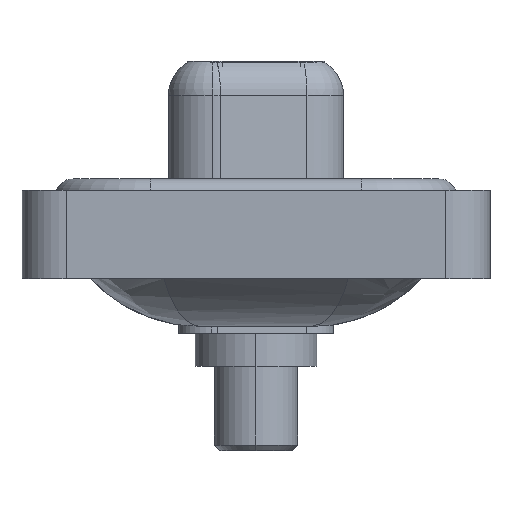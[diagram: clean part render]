
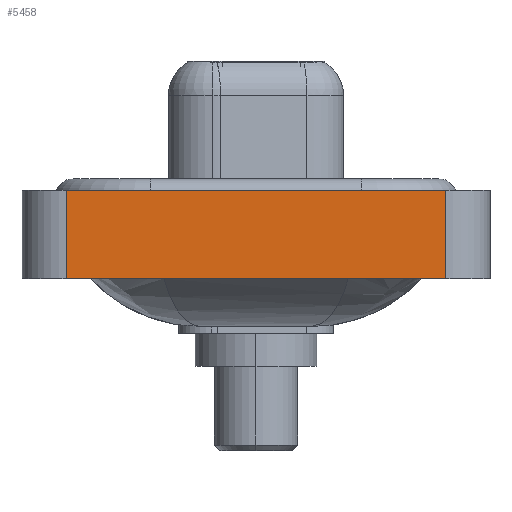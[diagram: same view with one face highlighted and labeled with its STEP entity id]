
A CAD part, left-side view. The second image highlights one B-rep face of the part: STEP entity #5458.
In plain terms, the highlighted planar face has unit normal (-1, 0, 0).
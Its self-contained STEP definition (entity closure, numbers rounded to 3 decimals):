
#371 = CARTESIAN_POINT ( 'NONE',  ( -7.35, -8.55, -3.6 ) ) ;
#1353 = CARTESIAN_POINT ( 'NONE',  ( -7.35, -8.55, 0.4 ) ) ;
#2004 = CARTESIAN_POINT ( 'NONE',  ( -7.35, 8.55, -3.6 ) ) ;
#2123 = CARTESIAN_POINT ( 'NONE',  ( -7.35, -8.55, -3.6 ) ) ;
#2218 = VERTEX_POINT ( 'NONE', #19889 ) ;
#2527 = ORIENTED_EDGE ( 'NONE', *, *, #4041, .T. ) ;
#3302 = ORIENTED_EDGE ( 'NONE', *, *, #20422, .F. ) ;
#3825 = LINE ( 'NONE', #2123, #8439 ) ;
#3907 = EDGE_CURVE ( 'NONE', #18494, #13088, #17138, .T. ) ;
#4041 = EDGE_CURVE ( 'NONE', #18494, #2218, #3825, .T. ) ;
#4106 = DIRECTION ( 'NONE',  ( 0., 0., 1. ) ) ;
#4123 = VECTOR ( 'NONE', #4106, 1000. ) ;
#4215 = VERTEX_POINT ( 'NONE', #6232 ) ;
#5009 = ORIENTED_EDGE ( 'NONE', *, *, #3907, .F. ) ;
#5226 = ORIENTED_EDGE ( 'NONE', *, *, #13923, .T. ) ;
#5458 = ADVANCED_FACE ( 'NONE', ( #18927 ), #20852, .T. ) ;
#5608 = CARTESIAN_POINT ( 'NONE',  ( -7.35, -8.55, -3.6 ) ) ;
#6232 = CARTESIAN_POINT ( 'NONE',  ( -7.35, -8.55, 0.4 ) ) ;
#6297 = VECTOR ( 'NONE', #21002, 1000. ) ;
#8290 = DIRECTION ( 'NONE',  ( 0., -1., 0. ) ) ;
#8439 = VECTOR ( 'NONE', #17816, 1000. ) ;
#9023 = LINE ( 'NONE', #5608, #4123 ) ;
#9526 = EDGE_LOOP ( 'NONE', ( #5226, #3302, #5009, #2527 ) ) ;
#9976 = AXIS2_PLACEMENT_3D ( 'NONE', #371, #15875, #14385 ) ;
#13088 = VERTEX_POINT ( 'NONE', #14495 ) ;
#13261 = CARTESIAN_POINT ( 'NONE',  ( -7.35, 8.55, -3.6 ) ) ;
#13923 = EDGE_CURVE ( 'NONE', #2218, #4215, #9023, .T. ) ;
#14385 = DIRECTION ( 'NONE',  ( 0., 0., 1. ) ) ;
#14495 = CARTESIAN_POINT ( 'NONE',  ( -7.35, 8.55, 0.4 ) ) ;
#14648 = VECTOR ( 'NONE', #8290, 1000. ) ;
#15875 = DIRECTION ( 'NONE',  ( -1., 0., 0. ) ) ;
#17138 = LINE ( 'NONE', #2004, #6297 ) ;
#17816 = DIRECTION ( 'NONE',  ( 0., -1., 0. ) ) ;
#18494 = VERTEX_POINT ( 'NONE', #13261 ) ;
#18927 = FACE_OUTER_BOUND ( 'NONE', #9526, .T. ) ;
#19889 = CARTESIAN_POINT ( 'NONE',  ( -7.35, -8.55, -3.6 ) ) ;
#20422 = EDGE_CURVE ( 'NONE', #13088, #4215, #20667, .T. ) ;
#20667 = LINE ( 'NONE', #1353, #14648 ) ;
#20852 = PLANE ( 'NONE',  #9976 ) ;
#21002 = DIRECTION ( 'NONE',  ( 0., 0., 1. ) ) ;
